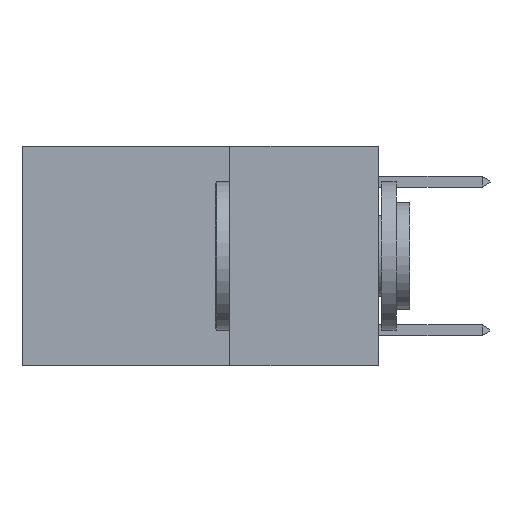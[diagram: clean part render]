
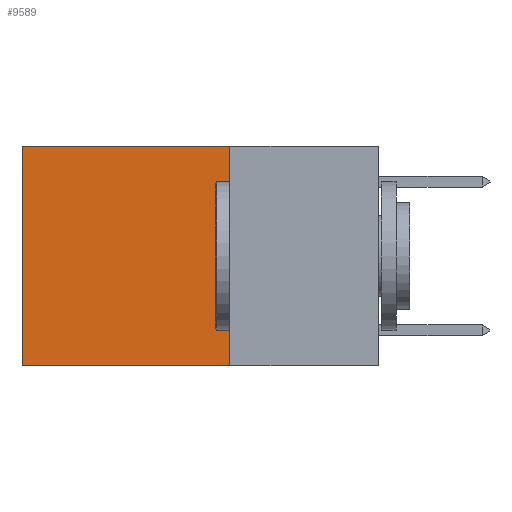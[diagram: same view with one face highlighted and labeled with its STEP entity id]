
A CAD part, left-side view. The second image highlights one B-rep face of the part: STEP entity #9589.
In plain terms, the highlighted planar face has unit normal (-1, 0, 0).
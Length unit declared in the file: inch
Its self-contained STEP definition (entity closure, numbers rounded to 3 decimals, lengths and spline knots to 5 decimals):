
#550 = VERTEX_POINT ( 'NONE', #9308 ) ;
#613 = DIRECTION ( 'NONE',  ( 1., 0., 0. ) ) ;
#1825 = CARTESIAN_POINT ( 'NONE',  ( 0.2625, 0.25, -0.37 ) ) ;
#1971 = LINE ( 'NONE', #1825, #11982 ) ;
#2767 = EDGE_CURVE ( 'NONE', #9239, #550, #4764, .T. ) ;
#3150 = EDGE_CURVE ( 'NONE', #9053, #4651, #4772, .T. ) ;
#4349 = DIRECTION ( 'NONE',  ( 0., 1., 0. ) ) ;
#4651 = VERTEX_POINT ( 'NONE', #13679 ) ;
#4687 = VECTOR ( 'NONE', #4349, 39.37008 ) ;
#4764 = LINE ( 'NONE', #8011, #5709 ) ;
#4772 = LINE ( 'NONE', #8016, #12842 ) ;
#5331 = DIRECTION ( 'NONE',  ( 0., 1., 0. ) ) ;
#5509 = ORIENTED_EDGE ( 'NONE', *, *, #3150, .F. ) ;
#5564 = LINE ( 'NONE', #8793, #4687 ) ;
#5709 = VECTOR ( 'NONE', #12367, 39.37008 ) ;
#6534 = EDGE_CURVE ( 'NONE', #4651, #550, #1971, .T. ) ;
#7617 = CARTESIAN_POINT ( 'NONE',  ( 0.2625, 0.6, 0. ) ) ;
#7937 = EDGE_CURVE ( 'NONE', #9053, #9239, #5564, .T. ) ;
#7974 = FACE_OUTER_BOUND ( 'NONE', #10019, .T. ) ;
#8011 = CARTESIAN_POINT ( 'NONE',  ( 0.2625, 0.6, 0. ) ) ;
#8016 = CARTESIAN_POINT ( 'NONE',  ( 0.2625, 0.25, 0. ) ) ;
#8793 = CARTESIAN_POINT ( 'NONE',  ( 0.2625, 0.25, 0. ) ) ;
#9053 = VERTEX_POINT ( 'NONE', #9757 ) ;
#9170 = PLANE ( 'NONE',  #10436 ) ;
#9239 = VERTEX_POINT ( 'NONE', #7617 ) ;
#9308 = CARTESIAN_POINT ( 'NONE',  ( 0.2625, 0.6, -0.37 ) ) ;
#9401 = DIRECTION ( 'NONE',  ( 0., 0., -1. ) ) ;
#9589 = ADVANCED_FACE ( 'NONE', ( #7974 ), #9170, .F. ) ;
#9757 = CARTESIAN_POINT ( 'NONE',  ( 0.2625, 0.25, 0. ) ) ;
#10019 = EDGE_LOOP ( 'NONE', ( #11591, #10525, #5509, #12915 ) ) ;
#10338 = CARTESIAN_POINT ( 'NONE',  ( 0.2625, 0.25, 0. ) ) ;
#10436 = AXIS2_PLACEMENT_3D ( 'NONE', #10338, #613, #9401 ) ;
#10525 = ORIENTED_EDGE ( 'NONE', *, *, #6534, .F. ) ;
#11591 = ORIENTED_EDGE ( 'NONE', *, *, #2767, .T. ) ;
#11982 = VECTOR ( 'NONE', #5331, 39.37008 ) ;
#12367 = DIRECTION ( 'NONE',  ( 0., 0., -1. ) ) ;
#12376 = DIRECTION ( 'NONE',  ( 0., 0., -1. ) ) ;
#12842 = VECTOR ( 'NONE', #12376, 39.37008 ) ;
#12915 = ORIENTED_EDGE ( 'NONE', *, *, #7937, .T. ) ;
#13679 = CARTESIAN_POINT ( 'NONE',  ( 0.2625, 0.25, -0.37 ) ) ;
